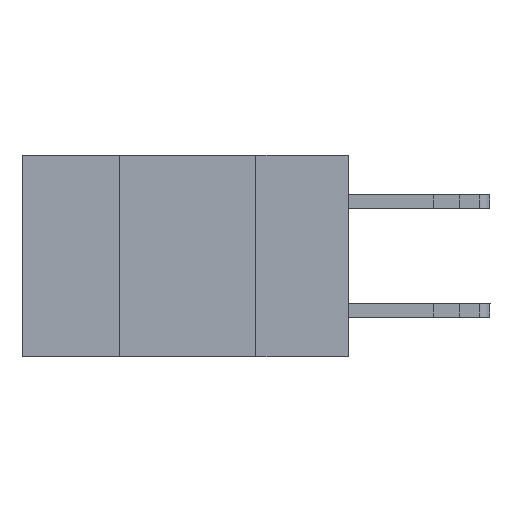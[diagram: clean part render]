
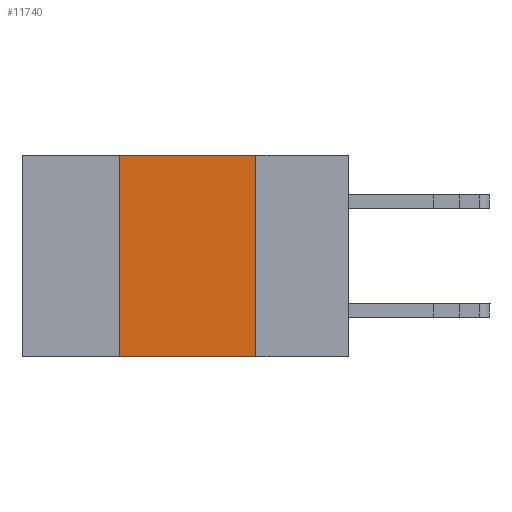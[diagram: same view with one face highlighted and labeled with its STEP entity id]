
A CAD part, left-side view. The second image highlights one B-rep face of the part: STEP entity #11740.
In plain terms, the highlighted planar face has unit normal (-1, 0, 0).
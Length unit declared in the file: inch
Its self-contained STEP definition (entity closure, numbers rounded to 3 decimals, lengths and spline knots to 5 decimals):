
#499 = CARTESIAN_POINT ( 'NONE',  ( 0., 0.42, 0. ) ) ;
#505 = DIRECTION ( 'NONE',  ( 0., -1., 0. ) ) ;
#702 = CARTESIAN_POINT ( 'NONE',  ( 0., 0.6, 0. ) ) ;
#804 = LINE ( 'NONE', #13045, #5721 ) ;
#1888 = CARTESIAN_POINT ( 'NONE',  ( 0., 0.17, -0.37 ) ) ;
#2049 = CARTESIAN_POINT ( 'NONE',  ( 0., 0.17, 0. ) ) ;
#2184 = DIRECTION ( 'NONE',  ( 0., 0., -1. ) ) ;
#2542 = VERTEX_POINT ( 'NONE', #8799 ) ;
#3537 = ORIENTED_EDGE ( 'NONE', *, *, #9940, .F. ) ;
#4499 = VERTEX_POINT ( 'NONE', #499 ) ;
#4703 = DIRECTION ( 'NONE',  ( 0., -1., 0. ) ) ;
#5036 = EDGE_CURVE ( 'NONE', #4499, #2542, #10979, .T. ) ;
#5082 = DIRECTION ( 'NONE',  ( 1., 0., 0. ) ) ;
#5721 = VECTOR ( 'NONE', #13458, 39.37008 ) ;
#6023 = CARTESIAN_POINT ( 'NONE',  ( 0., 0.6, -0.37 ) ) ;
#6200 = ORIENTED_EDGE ( 'NONE', *, *, #9535, .T. ) ;
#6204 = ORIENTED_EDGE ( 'NONE', *, *, #11168, .F. ) ;
#7101 = VECTOR ( 'NONE', #4703, 39.37008 ) ;
#7196 = ORIENTED_EDGE ( 'NONE', *, *, #5036, .F. ) ;
#7231 = EDGE_LOOP ( 'NONE', ( #3537, #7196, #6204, #6200 ) ) ;
#7781 = VERTEX_POINT ( 'NONE', #1888 ) ;
#8277 = VERTEX_POINT ( 'NONE', #13577 ) ;
#8799 = CARTESIAN_POINT ( 'NONE',  ( 0., 0.17, 0. ) ) ;
#9535 = EDGE_CURVE ( 'NONE', #8277, #7781, #13804, .T. ) ;
#9728 = FACE_OUTER_BOUND ( 'NONE', #7231, .T. ) ;
#9940 = EDGE_CURVE ( 'NONE', #2542, #7781, #10128, .T. ) ;
#10128 = LINE ( 'NONE', #2049, #13119 ) ;
#10978 = VECTOR ( 'NONE', #505, 39.37008 ) ;
#10979 = LINE ( 'NONE', #11124, #7101 ) ;
#11124 = CARTESIAN_POINT ( 'NONE',  ( 0., 0.6, 0. ) ) ;
#11168 = EDGE_CURVE ( 'NONE', #8277, #4499, #804, .T. ) ;
#11463 = PLANE ( 'NONE',  #12023 ) ;
#11740 = ADVANCED_FACE ( 'NONE', ( #9728 ), #11463, .F. ) ;
#11792 = DIRECTION ( 'NONE',  ( 0., 0., -1. ) ) ;
#12023 = AXIS2_PLACEMENT_3D ( 'NONE', #702, #5082, #11792 ) ;
#13045 = CARTESIAN_POINT ( 'NONE',  ( 0., 0.42, 0. ) ) ;
#13119 = VECTOR ( 'NONE', #2184, 39.37008 ) ;
#13458 = DIRECTION ( 'NONE',  ( 0., 0., 1. ) ) ;
#13577 = CARTESIAN_POINT ( 'NONE',  ( 0., 0.42, -0.37 ) ) ;
#13804 = LINE ( 'NONE', #6023, #10978 ) ;
